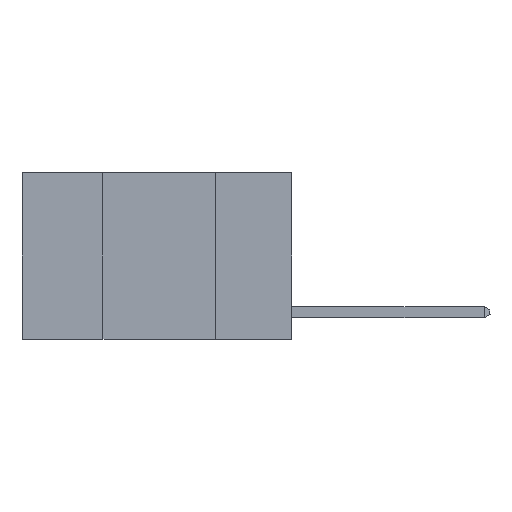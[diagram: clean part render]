
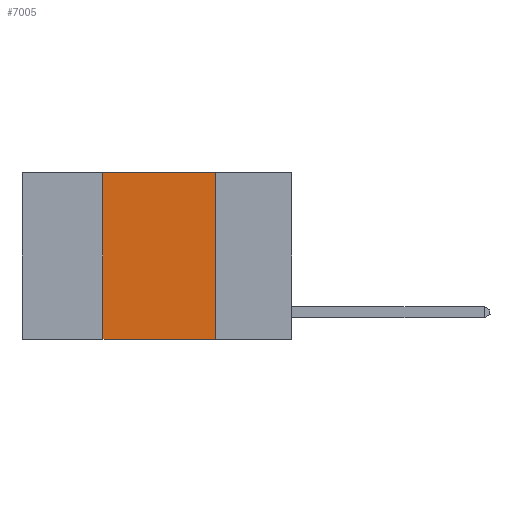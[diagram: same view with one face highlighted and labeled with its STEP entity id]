
A CAD part, left-side view. The second image highlights one B-rep face of the part: STEP entity #7005.
In plain terms, the highlighted planar face has unit normal (-1, 0, 0).
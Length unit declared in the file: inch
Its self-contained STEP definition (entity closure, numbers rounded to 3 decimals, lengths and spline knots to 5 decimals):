
#757 = CARTESIAN_POINT ( 'NONE',  ( 0., 0.6, -0.37 ) ) ;
#1576 = EDGE_CURVE ( 'NONE', #8657, #6599, #7865, .T. ) ;
#1902 = LINE ( 'NONE', #6522, #3129 ) ;
#2253 = LINE ( 'NONE', #4749, #3788 ) ;
#2370 = ORIENTED_EDGE ( 'NONE', *, *, #1576, .T. ) ;
#2598 = ORIENTED_EDGE ( 'NONE', *, *, #14792, .F. ) ;
#3129 = VECTOR ( 'NONE', #13513, 39.37008 ) ;
#3664 = CARTESIAN_POINT ( 'NONE',  ( 0., 0.17, 0. ) ) ;
#3788 = VECTOR ( 'NONE', #12958, 39.37008 ) ;
#3924 = VERTEX_POINT ( 'NONE', #3664 ) ;
#4639 = CARTESIAN_POINT ( 'NONE',  ( 0., 0.6, 0. ) ) ;
#4749 = CARTESIAN_POINT ( 'NONE',  ( 0., 0.17, 0. ) ) ;
#5242 = CARTESIAN_POINT ( 'NONE',  ( 0., 0.17, -0.37 ) ) ;
#5441 = VERTEX_POINT ( 'NONE', #7531 ) ;
#5726 = ORIENTED_EDGE ( 'NONE', *, *, #12236, .F. ) ;
#6008 = PLANE ( 'NONE',  #9948 ) ;
#6371 = ORIENTED_EDGE ( 'NONE', *, *, #9681, .F. ) ;
#6522 = CARTESIAN_POINT ( 'NONE',  ( 0., 0.6, 0. ) ) ;
#6599 = VERTEX_POINT ( 'NONE', #5242 ) ;
#6844 = FACE_OUTER_BOUND ( 'NONE', #13052, .T. ) ;
#7005 = ADVANCED_FACE ( 'NONE', ( #6844 ), #6008, .F. ) ;
#7531 = CARTESIAN_POINT ( 'NONE',  ( 0., 0.42, 0. ) ) ;
#7865 = LINE ( 'NONE', #757, #9274 ) ;
#8207 = DIRECTION ( 'NONE',  ( 1., 0., 0. ) ) ;
#8657 = VERTEX_POINT ( 'NONE', #11066 ) ;
#8936 = VECTOR ( 'NONE', #13292, 39.37008 ) ;
#9274 = VECTOR ( 'NONE', #10075, 39.37008 ) ;
#9681 = EDGE_CURVE ( 'NONE', #5441, #3924, #1902, .T. ) ;
#9948 = AXIS2_PLACEMENT_3D ( 'NONE', #4639, #8207, #10645 ) ;
#10075 = DIRECTION ( 'NONE',  ( 0., -1., 0. ) ) ;
#10645 = DIRECTION ( 'NONE',  ( 0., 0., -1. ) ) ;
#11010 = LINE ( 'NONE', #14264, #8936 ) ;
#11066 = CARTESIAN_POINT ( 'NONE',  ( 0., 0.42, -0.37 ) ) ;
#12236 = EDGE_CURVE ( 'NONE', #3924, #6599, #2253, .T. ) ;
#12958 = DIRECTION ( 'NONE',  ( 0., 0., -1. ) ) ;
#13052 = EDGE_LOOP ( 'NONE', ( #5726, #6371, #2598, #2370 ) ) ;
#13292 = DIRECTION ( 'NONE',  ( 0., 0., 1. ) ) ;
#13513 = DIRECTION ( 'NONE',  ( 0., -1., 0. ) ) ;
#14264 = CARTESIAN_POINT ( 'NONE',  ( 0., 0.42, 0. ) ) ;
#14792 = EDGE_CURVE ( 'NONE', #8657, #5441, #11010, .T. ) ;
